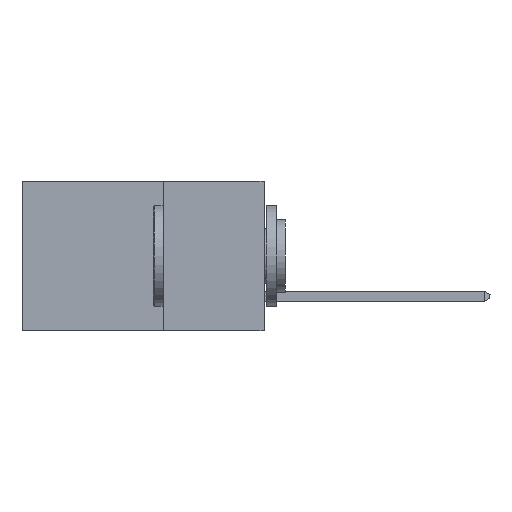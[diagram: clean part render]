
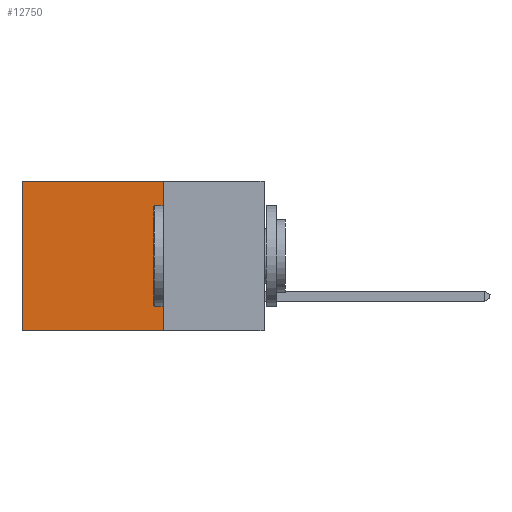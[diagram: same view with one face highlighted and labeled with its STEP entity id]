
A CAD part, left-side view. The second image highlights one B-rep face of the part: STEP entity #12750.
In plain terms, the highlighted planar face has unit normal (-1, 0, 0).
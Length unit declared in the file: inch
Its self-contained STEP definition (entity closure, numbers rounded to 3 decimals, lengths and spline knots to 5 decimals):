
#21 = AXIS2_PLACEMENT_3D ( 'NONE', #3950, #22989, #8692 ) ;
#332 = EDGE_CURVE ( 'NONE', #20340, #29631, #30594, .T. ) ;
#1761 = EDGE_LOOP ( 'NONE', ( #16580, #8663, #5324, #20166 ) ) ;
#1919 = VECTOR ( 'NONE', #24848, 39.37008 ) ;
#2841 = CARTESIAN_POINT ( 'NONE',  ( 0.298, 0.6, 0. ) ) ;
#3772 = DIRECTION ( 'NONE',  ( 0., 1., 0. ) ) ;
#3950 = CARTESIAN_POINT ( 'NONE',  ( 0.298, 0.25, 0. ) ) ;
#4250 = EDGE_CURVE ( 'NONE', #29631, #20018, #8240, .T. ) ;
#5324 = ORIENTED_EDGE ( 'NONE', *, *, #332, .F. ) ;
#8233 = LINE ( 'NONE', #10923, #20221 ) ;
#8240 = LINE ( 'NONE', #26151, #1919 ) ;
#8663 = ORIENTED_EDGE ( 'NONE', *, *, #4250, .F. ) ;
#8692 = DIRECTION ( 'NONE',  ( 0., 0., -1. ) ) ;
#8893 = FACE_OUTER_BOUND ( 'NONE', #1761, .T. ) ;
#10923 = CARTESIAN_POINT ( 'NONE',  ( 0.298, 0.25, 0. ) ) ;
#12750 = ADVANCED_FACE ( 'NONE', ( #8893 ), #20656, .F. ) ;
#13623 = CARTESIAN_POINT ( 'NONE',  ( 0.298, 0.25, 0. ) ) ;
#13758 = EDGE_CURVE ( 'NONE', #18815, #20018, #30293, .T. ) ;
#16345 = CARTESIAN_POINT ( 'NONE',  ( 0.298, 0.6, -0.37 ) ) ;
#16388 = CARTESIAN_POINT ( 'NONE',  ( 0.298, 0.25, -0.37 ) ) ;
#16580 = ORIENTED_EDGE ( 'NONE', *, *, #13758, .T. ) ;
#18178 = VECTOR ( 'NONE', #25367, 39.37008 ) ;
#18815 = VERTEX_POINT ( 'NONE', #19425 ) ;
#19425 = CARTESIAN_POINT ( 'NONE',  ( 0.298, 0.6, 0. ) ) ;
#20018 = VERTEX_POINT ( 'NONE', #16345 ) ;
#20166 = ORIENTED_EDGE ( 'NONE', *, *, #29486, .T. ) ;
#20221 = VECTOR ( 'NONE', #3772, 39.37008 ) ;
#20340 = VERTEX_POINT ( 'NONE', #27122 ) ;
#20656 = PLANE ( 'NONE',  #21 ) ;
#22989 = DIRECTION ( 'NONE',  ( 1., 0., 0. ) ) ;
#23380 = VECTOR ( 'NONE', #28902, 39.37008 ) ;
#24848 = DIRECTION ( 'NONE',  ( 0., 1., 0. ) ) ;
#25367 = DIRECTION ( 'NONE',  ( 0., 0., -1. ) ) ;
#26151 = CARTESIAN_POINT ( 'NONE',  ( 0.298, 0.25, -0.37 ) ) ;
#27122 = CARTESIAN_POINT ( 'NONE',  ( 0.298, 0.25, 0. ) ) ;
#28902 = DIRECTION ( 'NONE',  ( 0., 0., -1. ) ) ;
#29486 = EDGE_CURVE ( 'NONE', #20340, #18815, #8233, .T. ) ;
#29631 = VERTEX_POINT ( 'NONE', #16388 ) ;
#30293 = LINE ( 'NONE', #2841, #23380 ) ;
#30594 = LINE ( 'NONE', #13623, #18178 ) ;
